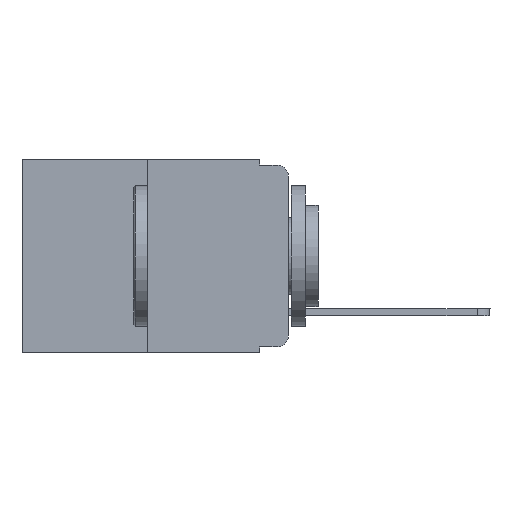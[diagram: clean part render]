
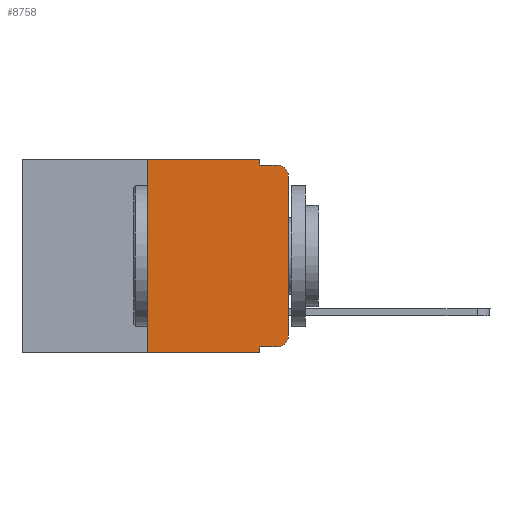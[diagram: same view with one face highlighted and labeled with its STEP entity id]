
A CAD part, left-side view. The second image highlights one B-rep face of the part: STEP entity #8758.
In plain terms, the highlighted planar face has unit normal (-1, 0, 0).
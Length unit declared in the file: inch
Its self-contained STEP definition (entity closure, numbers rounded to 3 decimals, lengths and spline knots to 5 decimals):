
#177 = VECTOR ( 'NONE', #5512, 39.37008 ) ;
#218 = EDGE_LOOP ( 'NONE', ( #8999, #11558, #6821, #1145, #12752, #578, #10005, #12290, #3902, #6433 ) ) ;
#370 = CARTESIAN_POINT ( 'NONE',  ( 0., 0.02, -0.313 ) ) ;
#392 = VECTOR ( 'NONE', #5079, 39.37008 ) ;
#489 = DIRECTION ( 'NONE',  ( 0., -1., 0. ) ) ;
#578 = ORIENTED_EDGE ( 'NONE', *, *, #4503, .F. ) ;
#708 = AXIS2_PLACEMENT_3D ( 'NONE', #370, #10154, #7293 ) ;
#941 = CARTESIAN_POINT ( 'NONE',  ( 0., 0.051, -0.333 ) ) ;
#1070 = VECTOR ( 'NONE', #9620, 39.37008 ) ;
#1145 = ORIENTED_EDGE ( 'NONE', *, *, #3436, .F. ) ;
#1179 = EDGE_CURVE ( 'NONE', #6699, #8471, #3831, .T. ) ;
#1504 = CARTESIAN_POINT ( 'NONE',  ( 0., 0.051, -0.01 ) ) ;
#1825 = VECTOR ( 'NONE', #489, 39.37008 ) ;
#2172 = LINE ( 'NONE', #12492, #1070 ) ;
#3002 = CIRCLE ( 'NONE', #10044, 0.02 ) ;
#3100 = CARTESIAN_POINT ( 'NONE',  ( 0., 0.02, -0.01 ) ) ;
#3362 = VERTEX_POINT ( 'NONE', #6643 ) ;
#3436 = EDGE_CURVE ( 'NONE', #12818, #6699, #2172, .T. ) ;
#3494 = LINE ( 'NONE', #11450, #7642 ) ;
#3767 = DIRECTION ( 'NONE',  ( 0., -1., 0. ) ) ;
#3831 = LINE ( 'NONE', #1504, #1825 ) ;
#3902 = ORIENTED_EDGE ( 'NONE', *, *, #10377, .T. ) ;
#3977 = CIRCLE ( 'NONE', #708, 0.02 ) ;
#4098 = CARTESIAN_POINT ( 'NONE',  ( 0., 0.02, -0.333 ) ) ;
#4123 = VERTEX_POINT ( 'NONE', #6987 ) ;
#4503 = EDGE_CURVE ( 'NONE', #11827, #4123, #12353, .T. ) ;
#4713 = CARTESIAN_POINT ( 'NONE',  ( 0., 0.473, 0. ) ) ;
#4952 = FACE_OUTER_BOUND ( 'NONE', #218, .T. ) ;
#5079 = DIRECTION ( 'NONE',  ( 0., -1., 0. ) ) ;
#5512 = DIRECTION ( 'NONE',  ( 0., 0., 1. ) ) ;
#5636 = LINE ( 'NONE', #10527, #177 ) ;
#5747 = DIRECTION ( 'NONE',  ( 0., 0., -1. ) ) ;
#5750 = DIRECTION ( 'NONE',  ( 0., -1., 0. ) ) ;
#6030 = VECTOR ( 'NONE', #5750, 39.37008 ) ;
#6047 = CARTESIAN_POINT ( 'NONE',  ( 0., 0.051, -0.343 ) ) ;
#6148 = LINE ( 'NONE', #8041, #392 ) ;
#6202 = CARTESIAN_POINT ( 'NONE',  ( 0., 0.25, 0. ) ) ;
#6235 = DIRECTION ( 'NONE',  ( -1., 0., 0. ) ) ;
#6433 = ORIENTED_EDGE ( 'NONE', *, *, #7299, .T. ) ;
#6643 = CARTESIAN_POINT ( 'NONE',  ( 0., 0., -0.03 ) ) ;
#6699 = VERTEX_POINT ( 'NONE', #7228 ) ;
#6726 = VECTOR ( 'NONE', #5747, 39.37008 ) ;
#6821 = ORIENTED_EDGE ( 'NONE', *, *, #1179, .F. ) ;
#6987 = CARTESIAN_POINT ( 'NONE',  ( 0., 0.25, 0. ) ) ;
#7228 = CARTESIAN_POINT ( 'NONE',  ( 0., 0.051, -0.01 ) ) ;
#7293 = DIRECTION ( 'NONE',  ( 0., 0., -1. ) ) ;
#7299 = EDGE_CURVE ( 'NONE', #11268, #9159, #3977, .T. ) ;
#7642 = VECTOR ( 'NONE', #3767, 39.37008 ) ;
#7886 = CARTESIAN_POINT ( 'NONE',  ( 0., 0.25, -0.343 ) ) ;
#8041 = CARTESIAN_POINT ( 'NONE',  ( 0., 0.473, -0.343 ) ) ;
#8146 = CARTESIAN_POINT ( 'NONE',  ( 0., 0., -0.313 ) ) ;
#8350 = CARTESIAN_POINT ( 'NONE',  ( 0., 0.051, 0. ) ) ;
#8471 = VERTEX_POINT ( 'NONE', #3100 ) ;
#8488 = CARTESIAN_POINT ( 'NONE',  ( 0., 0.051, 0. ) ) ;
#8494 = PLANE ( 'NONE',  #8810 ) ;
#8758 = ADVANCED_FACE ( 'NONE', ( #4952 ), #8494, .F. ) ;
#8810 = AXIS2_PLACEMENT_3D ( 'NONE', #4713, #9505, #11445 ) ;
#8868 = EDGE_CURVE ( 'NONE', #4123, #12818, #12664, .T. ) ;
#8957 = VERTEX_POINT ( 'NONE', #941 ) ;
#8999 = ORIENTED_EDGE ( 'NONE', *, *, #11462, .T. ) ;
#9011 = DIRECTION ( 'NONE',  ( 0., 0., 1. ) ) ;
#9159 = VERTEX_POINT ( 'NONE', #8146 ) ;
#9171 = LINE ( 'NONE', #8350, #6726 ) ;
#9505 = DIRECTION ( 'NONE',  ( 1., 0., 0. ) ) ;
#9589 = CARTESIAN_POINT ( 'NONE',  ( 0., 0.473, 0. ) ) ;
#9620 = DIRECTION ( 'NONE',  ( 0., 0., -1. ) ) ;
#9721 = VECTOR ( 'NONE', #9011, 39.37008 ) ;
#10005 = ORIENTED_EDGE ( 'NONE', *, *, #11930, .T. ) ;
#10044 = AXIS2_PLACEMENT_3D ( 'NONE', #12193, #6235, #10242 ) ;
#10154 = DIRECTION ( 'NONE',  ( -1., 0., 0. ) ) ;
#10242 = DIRECTION ( 'NONE',  ( 0., 0., -1. ) ) ;
#10377 = EDGE_CURVE ( 'NONE', #8957, #11268, #3494, .T. ) ;
#10527 = CARTESIAN_POINT ( 'NONE',  ( 0., 0., 0. ) ) ;
#10738 = EDGE_CURVE ( 'NONE', #3362, #8471, #3002, .T. ) ;
#10915 = EDGE_CURVE ( 'NONE', #8957, #11167, #9171, .T. ) ;
#11167 = VERTEX_POINT ( 'NONE', #6047 ) ;
#11268 = VERTEX_POINT ( 'NONE', #4098 ) ;
#11445 = DIRECTION ( 'NONE',  ( 0., 0., -1. ) ) ;
#11450 = CARTESIAN_POINT ( 'NONE',  ( 0., 0.051, -0.333 ) ) ;
#11462 = EDGE_CURVE ( 'NONE', #9159, #3362, #5636, .T. ) ;
#11558 = ORIENTED_EDGE ( 'NONE', *, *, #10738, .T. ) ;
#11827 = VERTEX_POINT ( 'NONE', #7886 ) ;
#11930 = EDGE_CURVE ( 'NONE', #11827, #11167, #6148, .T. ) ;
#12193 = CARTESIAN_POINT ( 'NONE',  ( 0., 0.02, -0.03 ) ) ;
#12290 = ORIENTED_EDGE ( 'NONE', *, *, #10915, .F. ) ;
#12353 = LINE ( 'NONE', #6202, #9721 ) ;
#12492 = CARTESIAN_POINT ( 'NONE',  ( 0., 0.051, 0. ) ) ;
#12664 = LINE ( 'NONE', #9589, #6030 ) ;
#12752 = ORIENTED_EDGE ( 'NONE', *, *, #8868, .F. ) ;
#12818 = VERTEX_POINT ( 'NONE', #8488 ) ;
